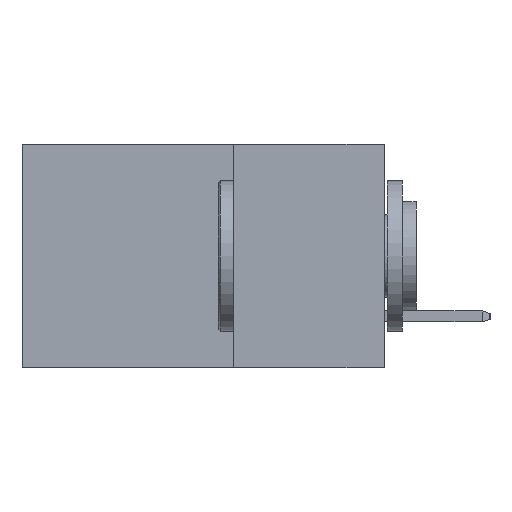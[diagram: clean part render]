
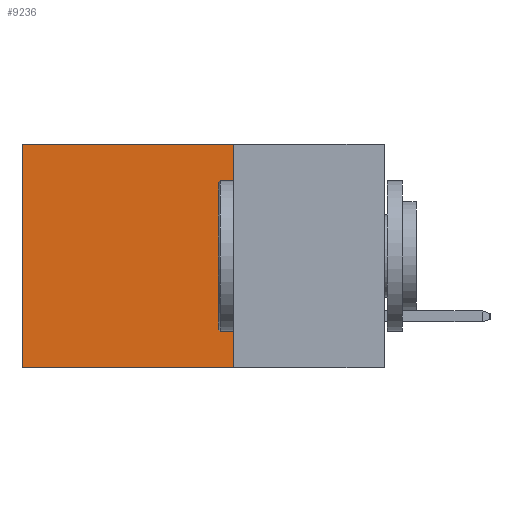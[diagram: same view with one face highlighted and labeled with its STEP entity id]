
A CAD part, left-side view. The second image highlights one B-rep face of the part: STEP entity #9236.
In plain terms, the highlighted planar face has unit normal (-1, 0, 0).
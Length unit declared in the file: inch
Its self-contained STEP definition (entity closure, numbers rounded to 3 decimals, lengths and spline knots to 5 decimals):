
#432 = VERTEX_POINT ( 'NONE', #11823 ) ;
#953 = VERTEX_POINT ( 'NONE', #15915 ) ;
#1383 = CARTESIAN_POINT ( 'NONE',  ( 0.2615, 0.6, 0. ) ) ;
#1484 = CARTESIAN_POINT ( 'NONE',  ( 0.2615, 0.6, -0.37 ) ) ;
#1665 = EDGE_CURVE ( 'NONE', #15153, #953, #3216, .T. ) ;
#1669 = DIRECTION ( 'NONE',  ( 0., 0., -1. ) ) ;
#2323 = DIRECTION ( 'NONE',  ( 0., 1., 0. ) ) ;
#2540 = DIRECTION ( 'NONE',  ( 0., 1., 0. ) ) ;
#2542 = CARTESIAN_POINT ( 'NONE',  ( 0.2615, 0.25, 0. ) ) ;
#2586 = VECTOR ( 'NONE', #11056, 39.37008 ) ;
#3216 = LINE ( 'NONE', #1484, #8007 ) ;
#3271 = LINE ( 'NONE', #12142, #7576 ) ;
#4288 = EDGE_CURVE ( 'NONE', #12149, #15153, #19793, .T. ) ;
#6075 = ORIENTED_EDGE ( 'NONE', *, *, #15973, .F. ) ;
#7052 = EDGE_LOOP ( 'NONE', ( #14453, #6075, #7282, #17744 ) ) ;
#7282 = ORIENTED_EDGE ( 'NONE', *, *, #11250, .F. ) ;
#7576 = VECTOR ( 'NONE', #2540, 39.37008 ) ;
#8007 = VECTOR ( 'NONE', #1669, 39.37008 ) ;
#9236 = ADVANCED_FACE ( 'NONE', ( #16174 ), #9512, .F. ) ;
#9346 = DIRECTION ( 'NONE',  ( 0., 0., -1. ) ) ;
#9387 = DIRECTION ( 'NONE',  ( 1., 0., 0. ) ) ;
#9470 = CARTESIAN_POINT ( 'NONE',  ( 0.2615, 0.25, -0.37 ) ) ;
#9512 = PLANE ( 'NONE',  #13618 ) ;
#10629 = LINE ( 'NONE', #20442, #2586 ) ;
#11056 = DIRECTION ( 'NONE',  ( 0., 0., -1. ) ) ;
#11250 = EDGE_CURVE ( 'NONE', #12149, #432, #10629, .T. ) ;
#11823 = CARTESIAN_POINT ( 'NONE',  ( 0.2615, 0.25, -0.37 ) ) ;
#12142 = CARTESIAN_POINT ( 'NONE',  ( 0.2615, 0.25, -0.37 ) ) ;
#12149 = VERTEX_POINT ( 'NONE', #19786 ) ;
#13618 = AXIS2_PLACEMENT_3D ( 'NONE', #9470, #9387, #9346 ) ;
#14453 = ORIENTED_EDGE ( 'NONE', *, *, #1665, .T. ) ;
#15153 = VERTEX_POINT ( 'NONE', #1383 ) ;
#15622 = VECTOR ( 'NONE', #2323, 39.37008 ) ;
#15915 = CARTESIAN_POINT ( 'NONE',  ( 0.2615, 0.6, -0.37 ) ) ;
#15973 = EDGE_CURVE ( 'NONE', #432, #953, #3271, .T. ) ;
#16174 = FACE_OUTER_BOUND ( 'NONE', #7052, .T. ) ;
#17744 = ORIENTED_EDGE ( 'NONE', *, *, #4288, .T. ) ;
#19786 = CARTESIAN_POINT ( 'NONE',  ( 0.2615, 0.25, 0. ) ) ;
#19793 = LINE ( 'NONE', #2542, #15622 ) ;
#20442 = CARTESIAN_POINT ( 'NONE',  ( 0.2615, 0.25, -0.37 ) ) ;
